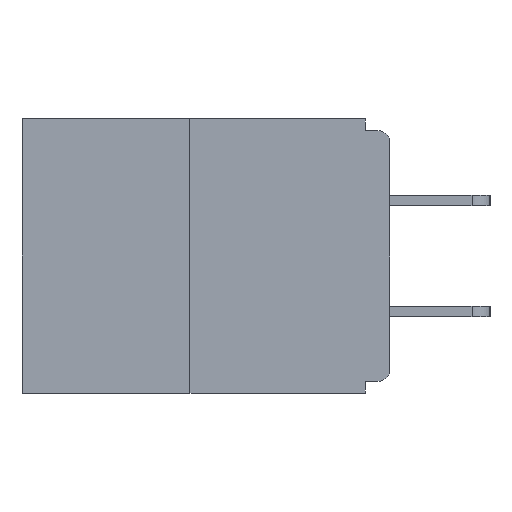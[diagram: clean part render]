
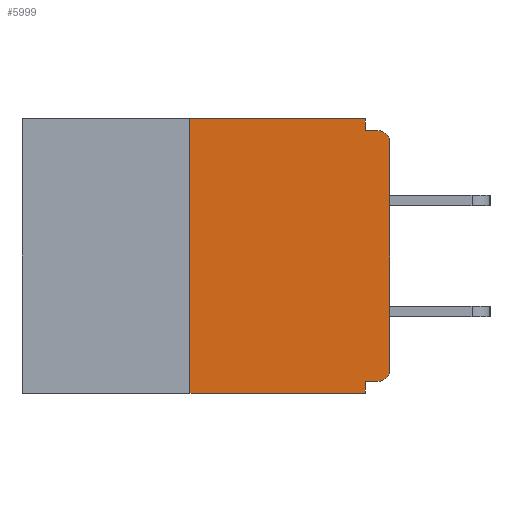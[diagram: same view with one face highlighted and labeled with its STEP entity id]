
A CAD part, left-side view. The second image highlights one B-rep face of the part: STEP entity #5999.
In plain terms, the highlighted planar face has unit normal (-1, 0, 0).
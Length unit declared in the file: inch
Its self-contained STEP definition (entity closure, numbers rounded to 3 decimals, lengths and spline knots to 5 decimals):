
#211 = DIRECTION ( 'NONE',  ( 0., 0., -1. ) ) ;
#727 = DIRECTION ( 'NONE',  ( -1., 0., 0. ) ) ;
#1362 = VECTOR ( 'NONE', #12238, 39.37008 ) ;
#1411 = VERTEX_POINT ( 'NONE', #13479 ) ;
#1473 = DIRECTION ( 'NONE',  ( 0., -1., 0. ) ) ;
#1578 = DIRECTION ( 'NONE',  ( 0., 0., -1. ) ) ;
#1717 = CARTESIAN_POINT ( 'NONE',  ( 0., 0., -0.313 ) ) ;
#1896 = CARTESIAN_POINT ( 'NONE',  ( 0., 0.031, -0.343 ) ) ;
#2626 = EDGE_CURVE ( 'NONE', #12913, #16202, #16238, .T. ) ;
#2821 = CARTESIAN_POINT ( 'NONE',  ( 0., 0.031, 0. ) ) ;
#2829 = EDGE_CURVE ( 'NONE', #12913, #4654, #6862, .T. ) ;
#2881 = CARTESIAN_POINT ( 'NONE',  ( 0., 0.46, 0. ) ) ;
#2915 = EDGE_LOOP ( 'NONE', ( #10719, #16907, #15626, #5825, #4528, #11390, #4272, #10342, #18673, #11037 ) ) ;
#2992 = CARTESIAN_POINT ( 'NONE',  ( 0., 0.25, -0.343 ) ) ;
#3153 = CARTESIAN_POINT ( 'NONE',  ( 0., 0., 0. ) ) ;
#3879 = LINE ( 'NONE', #2881, #11146 ) ;
#4036 = VECTOR ( 'NONE', #1578, 39.37008 ) ;
#4097 = EDGE_CURVE ( 'NONE', #14396, #7376, #8999, .T. ) ;
#4126 = EDGE_CURVE ( 'NONE', #16891, #14396, #12240, .T. ) ;
#4272 = ORIENTED_EDGE ( 'NONE', *, *, #5446, .T. ) ;
#4273 = CARTESIAN_POINT ( 'NONE',  ( 0., 0.25, 0. ) ) ;
#4326 = CARTESIAN_POINT ( 'NONE',  ( 0., 0.031, -0.343 ) ) ;
#4528 = ORIENTED_EDGE ( 'NONE', *, *, #8898, .F. ) ;
#4654 = VERTEX_POINT ( 'NONE', #1896 ) ;
#4869 = CARTESIAN_POINT ( 'NONE',  ( 0., 0., -0.03 ) ) ;
#5400 = DIRECTION ( 'NONE',  ( 0., 1., 0. ) ) ;
#5418 = LINE ( 'NONE', #8215, #14306 ) ;
#5446 = EDGE_CURVE ( 'NONE', #9261, #10487, #16120, .T. ) ;
#5533 = DIRECTION ( 'NONE',  ( 1., 0., 0. ) ) ;
#5825 = ORIENTED_EDGE ( 'NONE', *, *, #11572, .F. ) ;
#5999 = ADVANCED_FACE ( 'NONE', ( #12569 ), #12980, .F. ) ;
#6606 = CARTESIAN_POINT ( 'NONE',  ( 0., 0.015, -0.313 ) ) ;
#6633 = EDGE_CURVE ( 'NONE', #16202, #16891, #3879, .T. ) ;
#6716 = CARTESIAN_POINT ( 'NONE',  ( 0., 0.25, 0. ) ) ;
#6862 = LINE ( 'NONE', #7151, #14578 ) ;
#7151 = CARTESIAN_POINT ( 'NONE',  ( 0., 0.46, -0.343 ) ) ;
#7172 = CIRCLE ( 'NONE', #18670, 0.015 ) ;
#7376 = VERTEX_POINT ( 'NONE', #13127 ) ;
#7529 = DIRECTION ( 'NONE',  ( -1., 0., 0. ) ) ;
#7653 = VERTEX_POINT ( 'NONE', #16010 ) ;
#8117 = DIRECTION ( 'NONE',  ( 0., 0., -1. ) ) ;
#8215 = CARTESIAN_POINT ( 'NONE',  ( 0., 0., -0.328 ) ) ;
#8833 = DIRECTION ( 'NONE',  ( 0., 0., -1. ) ) ;
#8898 = EDGE_CURVE ( 'NONE', #1411, #7653, #5418, .T. ) ;
#8996 = DIRECTION ( 'NONE',  ( 0., -1., 0. ) ) ;
#8999 = LINE ( 'NONE', #16329, #17232 ) ;
#9261 = VERTEX_POINT ( 'NONE', #1717 ) ;
#10342 = ORIENTED_EDGE ( 'NONE', *, *, #17778, .T. ) ;
#10487 = VERTEX_POINT ( 'NONE', #4869 ) ;
#10719 = ORIENTED_EDGE ( 'NONE', *, *, #6633, .F. ) ;
#11037 = ORIENTED_EDGE ( 'NONE', *, *, #4126, .F. ) ;
#11146 = VECTOR ( 'NONE', #8996, 39.37008 ) ;
#11390 = ORIENTED_EDGE ( 'NONE', *, *, #15266, .T. ) ;
#11545 = AXIS2_PLACEMENT_3D ( 'NONE', #13390, #7529, #8833 ) ;
#11572 = EDGE_CURVE ( 'NONE', #7653, #4654, #12466, .T. ) ;
#12238 = DIRECTION ( 'NONE',  ( 0., 0., 1. ) ) ;
#12240 = LINE ( 'NONE', #18092, #13143 ) ;
#12466 = LINE ( 'NONE', #4326, #4036 ) ;
#12569 = FACE_OUTER_BOUND ( 'NONE', #2915, .T. ) ;
#12913 = VERTEX_POINT ( 'NONE', #2992 ) ;
#12980 = PLANE ( 'NONE',  #17135 ) ;
#13127 = CARTESIAN_POINT ( 'NONE',  ( 0., 0.015, -0.015 ) ) ;
#13143 = VECTOR ( 'NONE', #211, 39.37008 ) ;
#13390 = CARTESIAN_POINT ( 'NONE',  ( 0., 0.015, -0.03 ) ) ;
#13479 = CARTESIAN_POINT ( 'NONE',  ( 0., 0.015, -0.328 ) ) ;
#14306 = VECTOR ( 'NONE', #5400, 39.37008 ) ;
#14345 = CARTESIAN_POINT ( 'NONE',  ( 0., 0.46, 0. ) ) ;
#14396 = VERTEX_POINT ( 'NONE', #18351 ) ;
#14578 = VECTOR ( 'NONE', #19331, 39.37008 ) ;
#15266 = EDGE_CURVE ( 'NONE', #1411, #9261, #7172, .T. ) ;
#15626 = ORIENTED_EDGE ( 'NONE', *, *, #2829, .T. ) ;
#15999 = DIRECTION ( 'NONE',  ( 0., 0., -1. ) ) ;
#16010 = CARTESIAN_POINT ( 'NONE',  ( 0., 0.031, -0.328 ) ) ;
#16120 = LINE ( 'NONE', #3153, #1362 ) ;
#16202 = VERTEX_POINT ( 'NONE', #4273 ) ;
#16238 = LINE ( 'NONE', #6716, #16964 ) ;
#16329 = CARTESIAN_POINT ( 'NONE',  ( 0., 0., -0.015 ) ) ;
#16891 = VERTEX_POINT ( 'NONE', #2821 ) ;
#16907 = ORIENTED_EDGE ( 'NONE', *, *, #2626, .F. ) ;
#16964 = VECTOR ( 'NONE', #17324, 39.37008 ) ;
#17135 = AXIS2_PLACEMENT_3D ( 'NONE', #14345, #5533, #15999 ) ;
#17232 = VECTOR ( 'NONE', #1473, 39.37008 ) ;
#17324 = DIRECTION ( 'NONE',  ( 0., 0., 1. ) ) ;
#17682 = CIRCLE ( 'NONE', #11545, 0.015 ) ;
#17778 = EDGE_CURVE ( 'NONE', #10487, #7376, #17682, .T. ) ;
#18092 = CARTESIAN_POINT ( 'NONE',  ( 0., 0.031, 0. ) ) ;
#18351 = CARTESIAN_POINT ( 'NONE',  ( 0., 0.031, -0.015 ) ) ;
#18670 = AXIS2_PLACEMENT_3D ( 'NONE', #6606, #727, #8117 ) ;
#18673 = ORIENTED_EDGE ( 'NONE', *, *, #4097, .F. ) ;
#19331 = DIRECTION ( 'NONE',  ( 0., -1., 0. ) ) ;
